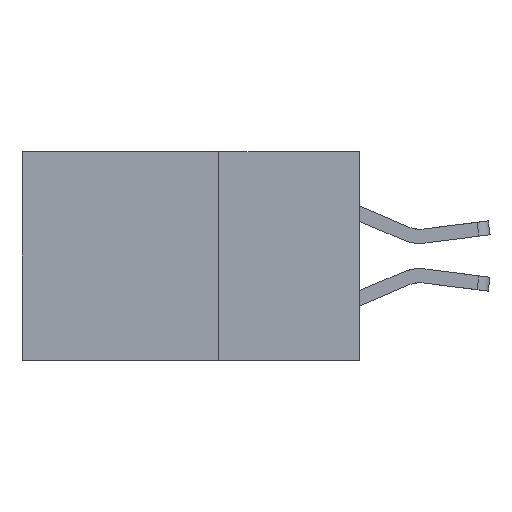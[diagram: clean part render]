
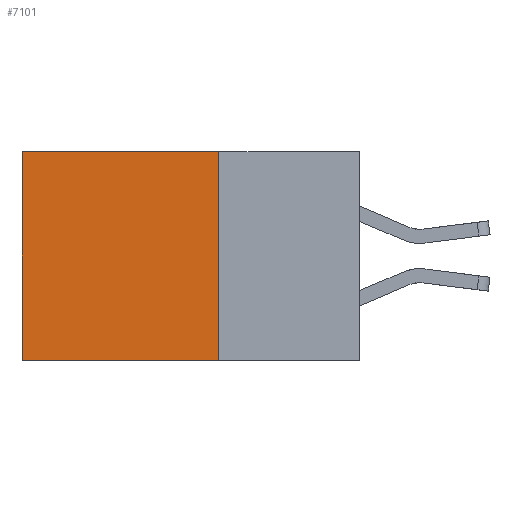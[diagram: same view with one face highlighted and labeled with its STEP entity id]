
A CAD part, left-side view. The second image highlights one B-rep face of the part: STEP entity #7101.
In plain terms, the highlighted planar face has unit normal (-1, 0, 0).
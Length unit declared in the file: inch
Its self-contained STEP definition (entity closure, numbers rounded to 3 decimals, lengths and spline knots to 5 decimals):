
#29 = FACE_OUTER_BOUND ( 'NONE', #13080, .T. ) ;
#188 = VECTOR ( 'NONE', #12998, 39.37008 ) ;
#519 = LINE ( 'NONE', #10359, #4694 ) ;
#1031 = CARTESIAN_POINT ( 'NONE',  ( 0.2875, 0.6, 0. ) ) ;
#1224 = VERTEX_POINT ( 'NONE', #3558 ) ;
#1259 = DIRECTION ( 'NONE',  ( 1., 0., 0. ) ) ;
#1439 = CARTESIAN_POINT ( 'NONE',  ( 0.2875, 0.25, 0. ) ) ;
#1576 = VERTEX_POINT ( 'NONE', #4197 ) ;
#1683 = VERTEX_POINT ( 'NONE', #1031 ) ;
#1842 = EDGE_CURVE ( 'NONE', #1683, #11535, #519, .T. ) ;
#2152 = CARTESIAN_POINT ( 'NONE',  ( 0.2875, 0.25, -0.37 ) ) ;
#2597 = EDGE_CURVE ( 'NONE', #1576, #11535, #5300, .T. ) ;
#3558 = CARTESIAN_POINT ( 'NONE',  ( 0.2875, 0.25, 0. ) ) ;
#4006 = DIRECTION ( 'NONE',  ( 0., 1., 0. ) ) ;
#4197 = CARTESIAN_POINT ( 'NONE',  ( 0.2875, 0.25, -0.37 ) ) ;
#4417 = CARTESIAN_POINT ( 'NONE',  ( 0.2875, 0.25, 0. ) ) ;
#4649 = VECTOR ( 'NONE', #7203, 39.37008 ) ;
#4694 = VECTOR ( 'NONE', #8190, 39.37008 ) ;
#5008 = ORIENTED_EDGE ( 'NONE', *, *, #6709, .T. ) ;
#5300 = LINE ( 'NONE', #2152, #188 ) ;
#5624 = DIRECTION ( 'NONE',  ( 0., 0., -1. ) ) ;
#6709 = EDGE_CURVE ( 'NONE', #1224, #1683, #6888, .T. ) ;
#6888 = LINE ( 'NONE', #1439, #12558 ) ;
#7101 = ADVANCED_FACE ( 'NONE', ( #29 ), #11091, .F. ) ;
#7203 = DIRECTION ( 'NONE',  ( 0., 0., -1. ) ) ;
#7473 = ORIENTED_EDGE ( 'NONE', *, *, #13255, .F. ) ;
#8190 = DIRECTION ( 'NONE',  ( 0., 0., -1. ) ) ;
#10359 = CARTESIAN_POINT ( 'NONE',  ( 0.2875, 0.6, 0. ) ) ;
#11091 = PLANE ( 'NONE',  #13497 ) ;
#11535 = VERTEX_POINT ( 'NONE', #12740 ) ;
#11746 = LINE ( 'NONE', #12757, #4649 ) ;
#11759 = ORIENTED_EDGE ( 'NONE', *, *, #1842, .T. ) ;
#12558 = VECTOR ( 'NONE', #4006, 39.37008 ) ;
#12740 = CARTESIAN_POINT ( 'NONE',  ( 0.2875, 0.6, -0.37 ) ) ;
#12757 = CARTESIAN_POINT ( 'NONE',  ( 0.2875, 0.25, 0. ) ) ;
#12998 = DIRECTION ( 'NONE',  ( 0., 1., 0. ) ) ;
#13080 = EDGE_LOOP ( 'NONE', ( #11759, #13583, #7473, #5008 ) ) ;
#13255 = EDGE_CURVE ( 'NONE', #1224, #1576, #11746, .T. ) ;
#13497 = AXIS2_PLACEMENT_3D ( 'NONE', #4417, #1259, #5624 ) ;
#13583 = ORIENTED_EDGE ( 'NONE', *, *, #2597, .F. ) ;
